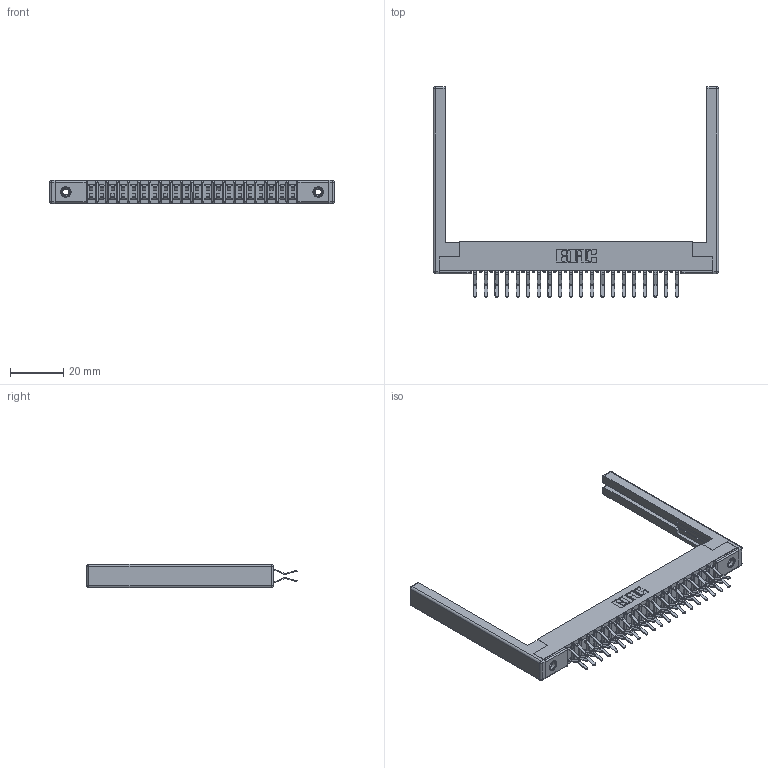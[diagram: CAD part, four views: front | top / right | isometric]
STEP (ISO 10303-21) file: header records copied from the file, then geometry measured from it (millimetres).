
FILE_DESCRIPTION (( 'STEP AP203' ), '1' );
FILE_NAME ('307-040-460-268.STEP', '2020-09-29T21:21:34', ( '' ), ( '' ), 'SwSTEP 2.0', 'SolidWorks 2020', '' );
FILE_SCHEMA (( 'CONFIG_CONTROL_DESIGN' ));
Length unit declared in the file: inch
Products named in the file (5): 307 Part_.156 Dia Mounting Holes; 307-290-001_560; 307-220-068; 307-040-460-268; 345-250-001_345-250-001-102
Assembly tree (45 placements, depth 2):
  307-040-460-268
    307 Part_.156 Dia Mounting Holes
    307-290-001_560  x40
    307-220-068  x2
    345-250-001_345-250-001-102  x2
Bounding box: 106.68 x 78.69 x 8.71 mm (x, y, z)
Volume: 11589.6 mm3; surface area: 16655.7 mm2
Topology: 45 solids, 45 shells, 2293 faces, 6393 edges, 4130 vertices
Faces by surface type: plane 1478, cylinder 749, sphere 50, cone 12, torus 4
Entity records: 23361 total; most frequent: CARTESIAN_POINT 3805, ORIENTED_EDGE 3760, DIRECTION 3752, EDGE_CURVE 1880, VECTOR 1430, LINE 1430, VERTEX_POINT 1214, AXIS2_PLACEMENT_3D 1161
